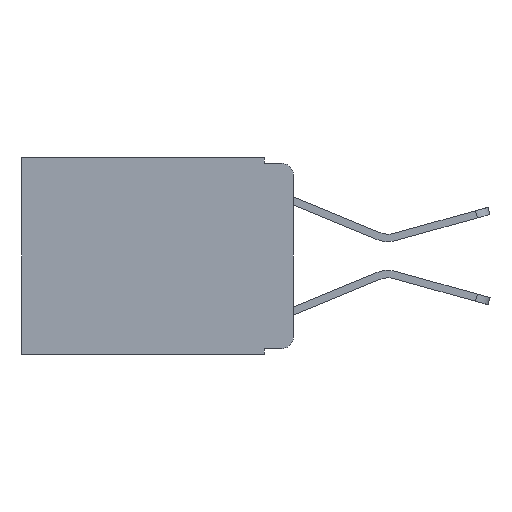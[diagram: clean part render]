
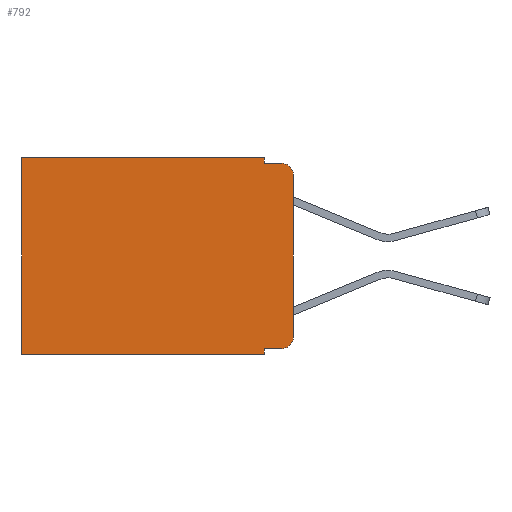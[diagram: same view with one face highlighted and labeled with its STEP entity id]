
A CAD part, left-side view. The second image highlights one B-rep face of the part: STEP entity #792.
In plain terms, the highlighted planar face has unit normal (-1, 0, 0).
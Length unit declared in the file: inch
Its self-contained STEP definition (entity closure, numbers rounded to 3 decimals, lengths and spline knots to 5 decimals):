
#489 = CARTESIAN_POINT ( 'NONE',  ( 0.298, 0., 0. ) ) ;
#592 = ORIENTED_EDGE ( 'NONE', *, *, #21126, .F. ) ;
#792 = ADVANCED_FACE ( 'NONE', ( #17136 ), #9896, .F. ) ;
#1256 = LINE ( 'NONE', #14049, #15574 ) ;
#1384 = LINE ( 'NONE', #12161, #5227 ) ;
#1648 = EDGE_CURVE ( 'NONE', #5532, #1761, #6318, .T. ) ;
#1761 = VERTEX_POINT ( 'NONE', #7054 ) ;
#2151 = CARTESIAN_POINT ( 'NONE',  ( 0.298, 0.051, 0. ) ) ;
#2170 = CARTESIAN_POINT ( 'NONE',  ( 0.298, 0.051, -0.343 ) ) ;
#2557 = DIRECTION ( 'NONE',  ( 0., 0., -1. ) ) ;
#2713 = CARTESIAN_POINT ( 'NONE',  ( 0.298, 0.051, 0. ) ) ;
#2932 = DIRECTION ( 'NONE',  ( 0., 0., -1. ) ) ;
#2955 = VERTEX_POINT ( 'NONE', #22123 ) ;
#3065 = EDGE_CURVE ( 'NONE', #3651, #1761, #1384, .T. ) ;
#3632 = DIRECTION ( 'NONE',  ( 0., -1., 0. ) ) ;
#3651 = VERTEX_POINT ( 'NONE', #11268 ) ;
#4792 = ORIENTED_EDGE ( 'NONE', *, *, #19083, .T. ) ;
#4977 = LINE ( 'NONE', #21891, #9369 ) ;
#5067 = CARTESIAN_POINT ( 'NONE',  ( 0.298, 0., -0.343 ) ) ;
#5227 = VECTOR ( 'NONE', #6499, 39.37008 ) ;
#5287 = ORIENTED_EDGE ( 'NONE', *, *, #10957, .F. ) ;
#5532 = VERTEX_POINT ( 'NONE', #5562 ) ;
#5548 = AXIS2_PLACEMENT_3D ( 'NONE', #6226, #13206, #11780 ) ;
#5562 = CARTESIAN_POINT ( 'NONE',  ( 0.298, 0.02, -0.333 ) ) ;
#5680 = VERTEX_POINT ( 'NONE', #2713 ) ;
#5860 = EDGE_LOOP ( 'NONE', ( #19576, #22907, #5287, #12802, #8866, #4792, #14200, #592, #9177, #19528 ) ) ;
#5893 = VERTEX_POINT ( 'NONE', #13844 ) ;
#6226 = CARTESIAN_POINT ( 'NONE',  ( 0.298, 0.02, -0.313 ) ) ;
#6318 = CIRCLE ( 'NONE', #5548, 0.02 ) ;
#6334 = CARTESIAN_POINT ( 'NONE',  ( 0.298, 0.02, -0.01 ) ) ;
#6499 = DIRECTION ( 'NONE',  ( 0., 0., -1. ) ) ;
#7054 = CARTESIAN_POINT ( 'NONE',  ( 0.298, 0., -0.313 ) ) ;
#7384 = CARTESIAN_POINT ( 'NONE',  ( 0.298, 0.473, -0.343 ) ) ;
#8075 = VERTEX_POINT ( 'NONE', #6334 ) ;
#8119 = DIRECTION ( 'NONE',  ( 1., 0., 0. ) ) ;
#8159 = VERTEX_POINT ( 'NONE', #7384 ) ;
#8486 = DIRECTION ( 'NONE',  ( 0., 1., 0. ) ) ;
#8866 = ORIENTED_EDGE ( 'NONE', *, *, #17986, .T. ) ;
#8913 = AXIS2_PLACEMENT_3D ( 'NONE', #22573, #8119, #2557 ) ;
#9177 = ORIENTED_EDGE ( 'NONE', *, *, #19756, .T. ) ;
#9241 = LINE ( 'NONE', #489, #10683 ) ;
#9369 = VECTOR ( 'NONE', #20354, 39.37008 ) ;
#9726 = CIRCLE ( 'NONE', #12751, 0.02 ) ;
#9896 = PLANE ( 'NONE',  #8913 ) ;
#10683 = VECTOR ( 'NONE', #16484, 39.37008 ) ;
#10957 = EDGE_CURVE ( 'NONE', #15969, #8075, #14303, .T. ) ;
#11243 = CARTESIAN_POINT ( 'NONE',  ( 0.298, 0.051, -0.333 ) ) ;
#11268 = CARTESIAN_POINT ( 'NONE',  ( 0.298, 0., -0.03 ) ) ;
#11408 = VECTOR ( 'NONE', #16389, 39.37008 ) ;
#11780 = DIRECTION ( 'NONE',  ( 0., 0., -1. ) ) ;
#12031 = DIRECTION ( 'NONE',  ( 0., 0., -1. ) ) ;
#12161 = CARTESIAN_POINT ( 'NONE',  ( 0.298, 0., 0. ) ) ;
#12751 = AXIS2_PLACEMENT_3D ( 'NONE', #23191, #23063, #2932 ) ;
#12802 = ORIENTED_EDGE ( 'NONE', *, *, #16903, .F. ) ;
#13206 = DIRECTION ( 'NONE',  ( -1., 0., 0. ) ) ;
#13844 = CARTESIAN_POINT ( 'NONE',  ( 0.298, 0.051, -0.333 ) ) ;
#14049 = CARTESIAN_POINT ( 'NONE',  ( 0.298, 0.473, 0. ) ) ;
#14200 = ORIENTED_EDGE ( 'NONE', *, *, #15913, .F. ) ;
#14303 = LINE ( 'NONE', #21527, #19316 ) ;
#14658 = VECTOR ( 'NONE', #8486, 39.37008 ) ;
#14682 = LINE ( 'NONE', #11243, #15596 ) ;
#15153 = DIRECTION ( 'NONE',  ( 0., -1., 0. ) ) ;
#15574 = VECTOR ( 'NONE', #12031, 39.37008 ) ;
#15596 = VECTOR ( 'NONE', #15153, 39.37008 ) ;
#15726 = CARTESIAN_POINT ( 'NONE',  ( 0.298, 0.051, -0.01 ) ) ;
#15848 = EDGE_CURVE ( 'NONE', #3651, #8075, #9726, .T. ) ;
#15913 = EDGE_CURVE ( 'NONE', #22714, #8159, #17517, .T. ) ;
#15969 = VERTEX_POINT ( 'NONE', #15726 ) ;
#16389 = DIRECTION ( 'NONE',  ( 0., 0., -1. ) ) ;
#16484 = DIRECTION ( 'NONE',  ( 0., 1., 0. ) ) ;
#16903 = EDGE_CURVE ( 'NONE', #5680, #15969, #4977, .T. ) ;
#17136 = FACE_OUTER_BOUND ( 'NONE', #5860, .T. ) ;
#17517 = LINE ( 'NONE', #5067, #14658 ) ;
#17986 = EDGE_CURVE ( 'NONE', #5680, #2955, #9241, .T. ) ;
#18379 = LINE ( 'NONE', #2151, #11408 ) ;
#19083 = EDGE_CURVE ( 'NONE', #2955, #8159, #1256, .T. ) ;
#19316 = VECTOR ( 'NONE', #3632, 39.37008 ) ;
#19528 = ORIENTED_EDGE ( 'NONE', *, *, #1648, .T. ) ;
#19576 = ORIENTED_EDGE ( 'NONE', *, *, #3065, .F. ) ;
#19756 = EDGE_CURVE ( 'NONE', #5893, #5532, #14682, .T. ) ;
#20354 = DIRECTION ( 'NONE',  ( 0., 0., -1. ) ) ;
#21126 = EDGE_CURVE ( 'NONE', #5893, #22714, #18379, .T. ) ;
#21527 = CARTESIAN_POINT ( 'NONE',  ( 0.298, 0.051, -0.01 ) ) ;
#21891 = CARTESIAN_POINT ( 'NONE',  ( 0.298, 0.051, 0. ) ) ;
#22123 = CARTESIAN_POINT ( 'NONE',  ( 0.298, 0.473, 0. ) ) ;
#22573 = CARTESIAN_POINT ( 'NONE',  ( 0.298, 0., 0. ) ) ;
#22714 = VERTEX_POINT ( 'NONE', #2170 ) ;
#22907 = ORIENTED_EDGE ( 'NONE', *, *, #15848, .T. ) ;
#23063 = DIRECTION ( 'NONE',  ( -1., 0., 0. ) ) ;
#23191 = CARTESIAN_POINT ( 'NONE',  ( 0.298, 0.02, -0.03 ) ) ;
